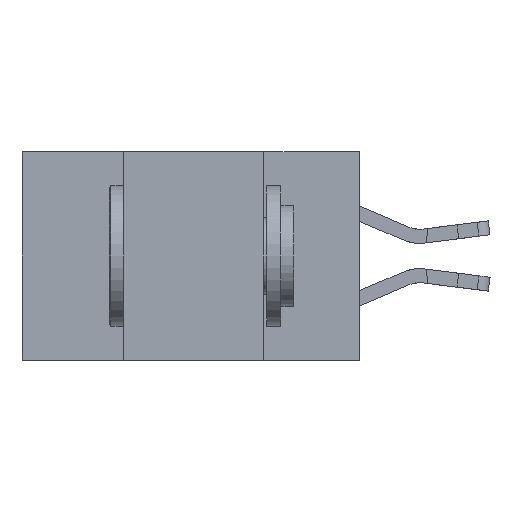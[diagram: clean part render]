
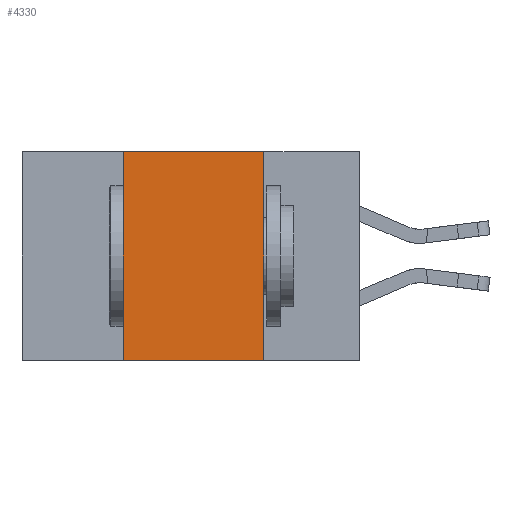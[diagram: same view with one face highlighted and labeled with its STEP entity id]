
A CAD part, left-side view. The second image highlights one B-rep face of the part: STEP entity #4330.
In plain terms, the highlighted planar face has unit normal (-1, 0, 0).
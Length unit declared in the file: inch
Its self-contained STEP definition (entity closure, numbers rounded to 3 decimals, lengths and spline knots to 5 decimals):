
#59 = EDGE_CURVE ( 'NONE', #9641, #18921, #6771, .T. ) ;
#401 = DIRECTION ( 'NONE',  ( 1., 0., 0. ) ) ;
#674 = VECTOR ( 'NONE', #20167, 39.37008 ) ;
#692 = VECTOR ( 'NONE', #22695, 39.37008 ) ;
#1426 = CARTESIAN_POINT ( 'NONE',  ( 0., 0.6, -0.37 ) ) ;
#1673 = ORIENTED_EDGE ( 'NONE', *, *, #10302, .T. ) ;
#1971 = VERTEX_POINT ( 'NONE', #19227 ) ;
#4330 = ADVANCED_FACE ( 'NONE', ( #11509 ), #11489, .F. ) ;
#5156 = DIRECTION ( 'NONE',  ( 0., -1., 0. ) ) ;
#5603 = LINE ( 'NONE', #14678, #674 ) ;
#6127 = VERTEX_POINT ( 'NONE', #17560 ) ;
#6771 = LINE ( 'NONE', #17365, #692 ) ;
#7796 = LINE ( 'NONE', #1426, #16381 ) ;
#8285 = EDGE_CURVE ( 'NONE', #1971, #9641, #20677, .T. ) ;
#8986 = CARTESIAN_POINT ( 'NONE',  ( 0., 0.42, 0. ) ) ;
#9208 = ORIENTED_EDGE ( 'NONE', *, *, #21073, .F. ) ;
#9641 = VERTEX_POINT ( 'NONE', #8986 ) ;
#10302 = EDGE_CURVE ( 'NONE', #1971, #6127, #7796, .T. ) ;
#11022 = VECTOR ( 'NONE', #21907, 39.37008 ) ;
#11489 = PLANE ( 'NONE',  #18174 ) ;
#11509 = FACE_OUTER_BOUND ( 'NONE', #21678, .T. ) ;
#13307 = DIRECTION ( 'NONE',  ( 0., 0., -1. ) ) ;
#14642 = ORIENTED_EDGE ( 'NONE', *, *, #8285, .F. ) ;
#14678 = CARTESIAN_POINT ( 'NONE',  ( 0., 0.17, 0. ) ) ;
#15900 = CARTESIAN_POINT ( 'NONE',  ( 0., 0.17, 0. ) ) ;
#16381 = VECTOR ( 'NONE', #5156, 39.37008 ) ;
#17365 = CARTESIAN_POINT ( 'NONE',  ( 0., 0.6, 0. ) ) ;
#17560 = CARTESIAN_POINT ( 'NONE',  ( 0., 0.17, -0.37 ) ) ;
#18174 = AXIS2_PLACEMENT_3D ( 'NONE', #22322, #401, #13307 ) ;
#18343 = CARTESIAN_POINT ( 'NONE',  ( 0., 0.42, 0. ) ) ;
#18921 = VERTEX_POINT ( 'NONE', #15900 ) ;
#19227 = CARTESIAN_POINT ( 'NONE',  ( 0., 0.42, -0.37 ) ) ;
#20167 = DIRECTION ( 'NONE',  ( 0., 0., -1. ) ) ;
#20677 = LINE ( 'NONE', #18343, #11022 ) ;
#21073 = EDGE_CURVE ( 'NONE', #18921, #6127, #5603, .T. ) ;
#21678 = EDGE_LOOP ( 'NONE', ( #9208, #23667, #14642, #1673 ) ) ;
#21907 = DIRECTION ( 'NONE',  ( 0., 0., 1. ) ) ;
#22322 = CARTESIAN_POINT ( 'NONE',  ( 0., 0.6, 0. ) ) ;
#22695 = DIRECTION ( 'NONE',  ( 0., -1., 0. ) ) ;
#23667 = ORIENTED_EDGE ( 'NONE', *, *, #59, .F. ) ;
